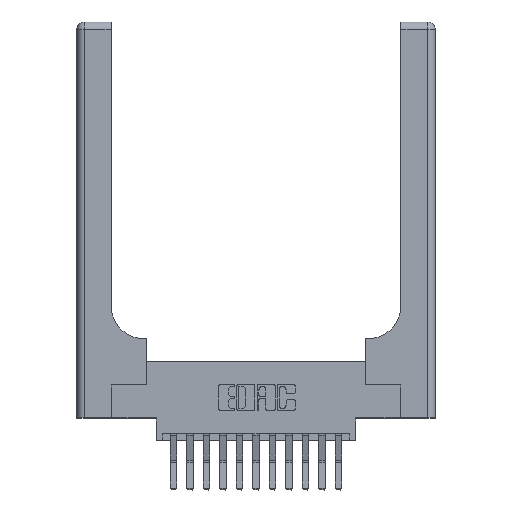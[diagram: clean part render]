
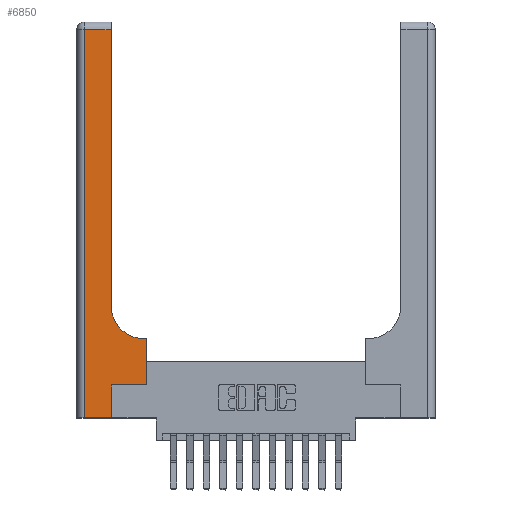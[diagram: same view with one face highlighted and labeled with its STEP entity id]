
A CAD part, top view. The second image highlights one B-rep face of the part: STEP entity #6850.
In plain terms, the highlighted planar face has unit normal (0, 0, 1).
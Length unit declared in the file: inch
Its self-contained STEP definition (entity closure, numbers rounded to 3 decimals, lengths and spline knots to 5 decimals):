
#72 = DIRECTION ( 'NONE',  ( 0., 1., 0. ) ) ;
#725 = CARTESIAN_POINT ( 'NONE',  ( 0., 2.94, 0.37 ) ) ;
#907 = EDGE_CURVE ( 'NONE', #10459, #2457, #8009, .T. ) ;
#1028 = ORIENTED_EDGE ( 'NONE', *, *, #907, .T. ) ;
#1523 = CARTESIAN_POINT ( 'NONE',  ( 0.26, 3., 0.37 ) ) ;
#2089 = CARTESIAN_POINT ( 'NONE',  ( 0.528, 0.25, 0.37 ) ) ;
#2457 = VERTEX_POINT ( 'NONE', #5775 ) ;
#2625 = FACE_OUTER_BOUND ( 'NONE', #12275, .T. ) ;
#2713 = EDGE_CURVE ( 'NONE', #10546, #13272, #4993, .T. ) ;
#2981 = AXIS2_PLACEMENT_3D ( 'NONE', #15819, #3890, #7983 ) ;
#3146 = VERTEX_POINT ( 'NONE', #3388 ) ;
#3388 = CARTESIAN_POINT ( 'NONE',  ( 0.26, 2.94, 0.37 ) ) ;
#3583 = CARTESIAN_POINT ( 'NONE',  ( 0.06, 2.94, 0.37 ) ) ;
#3661 = CARTESIAN_POINT ( 'NONE',  ( 0.265, 0., 0.37 ) ) ;
#3730 = CARTESIAN_POINT ( 'NONE',  ( 0.06, 0., 0.37 ) ) ;
#3841 = DIRECTION ( 'NONE',  ( 0., 1., 0. ) ) ;
#3890 = DIRECTION ( 'NONE',  ( 0., 0., -1. ) ) ;
#4095 = CARTESIAN_POINT ( 'NONE',  ( 0.26, 0.85, 0.37 ) ) ;
#4141 = ORIENTED_EDGE ( 'NONE', *, *, #12362, .T. ) ;
#4215 = CARTESIAN_POINT ( 'NONE',  ( 0., 3., 0.37 ) ) ;
#4635 = CARTESIAN_POINT ( 'NONE',  ( 0.265, 0.25, 0.37 ) ) ;
#4740 = CARTESIAN_POINT ( 'NONE',  ( 0.06, 3., 0.37 ) ) ;
#4822 = LINE ( 'NONE', #2089, #14064 ) ;
#4993 = LINE ( 'NONE', #4740, #13530 ) ;
#5060 = VERTEX_POINT ( 'NONE', #7591 ) ;
#5122 = CARTESIAN_POINT ( 'NONE',  ( 0.26, 0.6, 0.37 ) ) ;
#5334 = DIRECTION ( 'NONE',  ( 0., 0., -1. ) ) ;
#5755 = VECTOR ( 'NONE', #14585, 39.37008 ) ;
#5775 = CARTESIAN_POINT ( 'NONE',  ( 0.265, 0.25, 0.37 ) ) ;
#6034 = ORIENTED_EDGE ( 'NONE', *, *, #8825, .T. ) ;
#6047 = VERTEX_POINT ( 'NONE', #8125 ) ;
#6605 = ORIENTED_EDGE ( 'NONE', *, *, #12943, .T. ) ;
#6850 = ADVANCED_FACE ( 'NONE', ( #2625 ), #7003, .F. ) ;
#7003 = PLANE ( 'NONE',  #14286 ) ;
#7394 = VERTEX_POINT ( 'NONE', #4095 ) ;
#7591 = CARTESIAN_POINT ( 'NONE',  ( 0.528, 0.25, 0.37 ) ) ;
#7595 = DIRECTION ( 'NONE',  ( -1., 0., 0. ) ) ;
#7983 = DIRECTION ( 'NONE',  ( 1., 0., 0. ) ) ;
#8009 = LINE ( 'NONE', #13288, #16214 ) ;
#8125 = CARTESIAN_POINT ( 'NONE',  ( 0.51, 0.6, 0.37 ) ) ;
#8257 = VECTOR ( 'NONE', #12524, 39.37008 ) ;
#8400 = EDGE_CURVE ( 'NONE', #3146, #10546, #12626, .T. ) ;
#8591 = DIRECTION ( 'NONE',  ( 0., -1., 0. ) ) ;
#8606 = VECTOR ( 'NONE', #7595, 39.37008 ) ;
#8661 = LINE ( 'NONE', #4635, #8257 ) ;
#8695 = EDGE_CURVE ( 'NONE', #2457, #5060, #8661, .T. ) ;
#8825 = EDGE_CURVE ( 'NONE', #5060, #11076, #4822, .T. ) ;
#9430 = EDGE_CURVE ( 'NONE', #13272, #10459, #13445, .T. ) ;
#10459 = VERTEX_POINT ( 'NONE', #3661 ) ;
#10488 = CIRCLE ( 'NONE', #2981, 0.25 ) ;
#10546 = VERTEX_POINT ( 'NONE', #3583 ) ;
#10825 = DIRECTION ( 'NONE',  ( -1., 0., 0. ) ) ;
#11076 = VERTEX_POINT ( 'NONE', #12466 ) ;
#11224 = ORIENTED_EDGE ( 'NONE', *, *, #8695, .T. ) ;
#11471 = ORIENTED_EDGE ( 'NONE', *, *, #2713, .T. ) ;
#11480 = LINE ( 'NONE', #5122, #8606 ) ;
#11939 = EDGE_CURVE ( 'NONE', #7394, #3146, #15836, .T. ) ;
#12132 = VECTOR ( 'NONE', #15914, 39.37008 ) ;
#12275 = EDGE_LOOP ( 'NONE', ( #16979, #13671, #11471, #13613, #1028, #11224, #6034, #6605, #4141 ) ) ;
#12362 = EDGE_CURVE ( 'NONE', #6047, #7394, #10488, .T. ) ;
#12466 = CARTESIAN_POINT ( 'NONE',  ( 0.528, 0.6, 0.37 ) ) ;
#12524 = DIRECTION ( 'NONE',  ( 1., 0., 0. ) ) ;
#12544 = DIRECTION ( 'NONE',  ( -1., 0., 0. ) ) ;
#12626 = LINE ( 'NONE', #725, #16282 ) ;
#12943 = EDGE_CURVE ( 'NONE', #11076, #6047, #11480, .T. ) ;
#13168 = CARTESIAN_POINT ( 'NONE',  ( 0., 0., 0.37 ) ) ;
#13272 = VERTEX_POINT ( 'NONE', #3730 ) ;
#13288 = CARTESIAN_POINT ( 'NONE',  ( 0.265, 0., 0.37 ) ) ;
#13445 = LINE ( 'NONE', #13168, #5755 ) ;
#13530 = VECTOR ( 'NONE', #8591, 39.37008 ) ;
#13613 = ORIENTED_EDGE ( 'NONE', *, *, #9430, .T. ) ;
#13671 = ORIENTED_EDGE ( 'NONE', *, *, #8400, .T. ) ;
#14064 = VECTOR ( 'NONE', #3841, 39.37008 ) ;
#14286 = AXIS2_PLACEMENT_3D ( 'NONE', #4215, #5334, #10825 ) ;
#14585 = DIRECTION ( 'NONE',  ( 1., 0., 0. ) ) ;
#15819 = CARTESIAN_POINT ( 'NONE',  ( 0.51, 0.85, 0.37 ) ) ;
#15836 = LINE ( 'NONE', #1523, #12132 ) ;
#15914 = DIRECTION ( 'NONE',  ( 0., 1., 0. ) ) ;
#16214 = VECTOR ( 'NONE', #72, 39.37008 ) ;
#16282 = VECTOR ( 'NONE', #12544, 39.37008 ) ;
#16979 = ORIENTED_EDGE ( 'NONE', *, *, #11939, .T. ) ;
